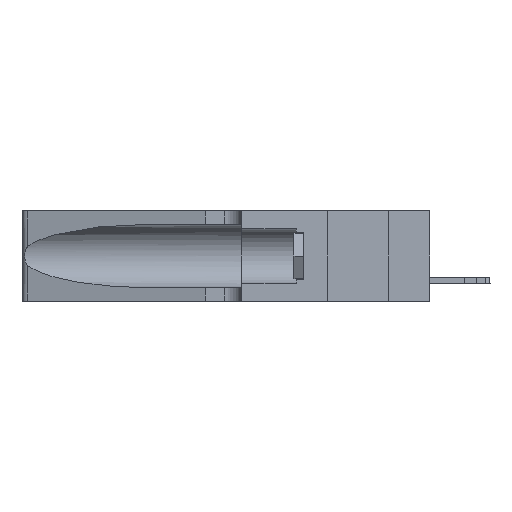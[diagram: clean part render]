
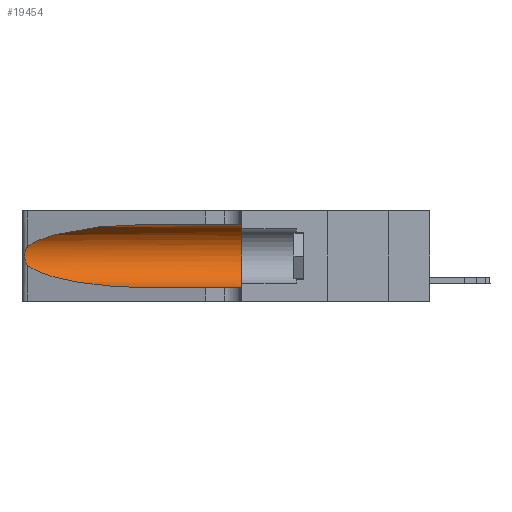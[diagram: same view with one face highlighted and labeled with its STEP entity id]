
A CAD part, left-side view. The second image highlights one B-rep face of the part: STEP entity #19454.
In plain terms, the highlighted cylindrical face has radius 3.308 mm (diameter 6.617 mm), a partial arc.
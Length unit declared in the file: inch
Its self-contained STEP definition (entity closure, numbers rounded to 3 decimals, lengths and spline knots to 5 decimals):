
#487 = ORIENTED_EDGE ( 'NONE', *, *, #19606, .T. ) ;
#594 = CARTESIAN_POINT ( 'NONE',  ( 0.1305, 0.72297, 0.05475 ) ) ;
#696 = CARTESIAN_POINT ( 'NONE',  ( 0.25854, 1.2359, 0.20912 ) ) ;
#829 = CARTESIAN_POINT ( 'NONE',  ( 0.25789, 1.23486, 0.15765 ) ) ;
#889 = CARTESIAN_POINT ( 'NONE',  ( 0.26075, 1.23896, 0.19203 ) ) ;
#1236 = DIRECTION ( 'NONE',  ( 0., -1., 0. ) ) ;
#1307 = DIRECTION ( 'NONE',  ( 0., 1., 0. ) ) ;
#1852 = EDGE_CURVE ( 'NONE', #2309, #6942, #5154, .T. ) ;
#2156 = EDGE_CURVE ( 'NONE', #19554, #5370, #11782, .T. ) ;
#2194 = CARTESIAN_POINT ( 'NONE',  ( 0.2373, 1.15595, 0.28018 ) ) ;
#2309 = VERTEX_POINT ( 'NONE', #5641 ) ;
#2811 = DIRECTION ( 'NONE',  ( 0., 0., -1. ) ) ;
#2937 = CARTESIAN_POINT ( 'NONE',  ( 0.25487, 1.22718, 0.14631 ) ) ;
#3590 = CARTESIAN_POINT ( 'NONE',  ( 0.25555, 1.22994, 0.2215 ) ) ;
#3851 = CARTESIAN_POINT ( 'NONE',  ( 0.26075, 1.23896, 0.178 ) ) ;
#3909 = VERTEX_POINT ( 'NONE', #14262 ) ;
#4840 = EDGE_LOOP ( 'NONE', ( #18273, #14750, #487, #16768, #6416, #5455 ) ) ;
#5136 = EDGE_CURVE ( 'NONE', #5370, #11224, #10935, .T. ) ;
#5154 = CIRCLE ( 'NONE', #13171, 0.13025 ) ;
#5287 = EDGE_CURVE ( 'NONE', #3909, #6942, #15941, .T. ) ;
#5370 = VERTEX_POINT ( 'NONE', #14126 ) ;
#5439 = CARTESIAN_POINT ( 'NONE',  ( 0.25787, 1.23484, 0.2124 ) ) ;
#5455 = ORIENTED_EDGE ( 'NONE', *, *, #14140, .F. ) ;
#5641 = CARTESIAN_POINT ( 'NONE',  ( 0.1305, 0.35, 0.31525 ) ) ;
#6026 = LINE ( 'NONE', #6101, #10466 ) ;
#6101 = CARTESIAN_POINT ( 'NONE',  ( 0.1305, 1.61858, 0.31525 ) ) ;
#6416 = ORIENTED_EDGE ( 'NONE', *, *, #1852, .F. ) ;
#6942 = VERTEX_POINT ( 'NONE', #18145 ) ;
#7665 = DIRECTION ( 'NONE',  ( 0., -1., 0. ) ) ;
#8390 = AXIS2_PLACEMENT_3D ( 'NONE', #10676, #1236, #2811 ) ;
#8391 = CARTESIAN_POINT ( 'NONE',  ( 0.18966, 0.96281, 0.31525 ) ) ;
#8731 = CARTESIAN_POINT ( 'NONE',  ( 0.1305, 0.72297, 0.31525 ) ) ;
#8964 = CARTESIAN_POINT ( 'NONE',  ( 0.1305, 0.35, 0.185 ) ) ;
#8981 = FACE_OUTER_BOUND ( 'NONE', #4840, .T. ) ;
#9329 = CARTESIAN_POINT ( 'NONE',  ( 0.1305, 1.61858, 0.05475 ) ) ;
#10265 = CARTESIAN_POINT ( 'NONE',  ( 0.25555, 1.22993, 0.14849 ) ) ;
#10466 = VECTOR ( 'NONE', #7665, 39.37008 ) ;
#10676 = CARTESIAN_POINT ( 'NONE',  ( 0.1305, 1.61858, 0.185 ) ) ;
#10935 = B_SPLINE_CURVE_WITH_KNOTS ( 'NONE', 3,
 ( #12938, #3590, #16096, #5439, #696, #14846, #889, #3851, #19593, #11866, #829, #16279, #10265, #16410 ),
 .UNSPECIFIED., .F., .F.,
 ( 4, 2, 2, 2, 2, 2, 4 ),
 ( 0., 0.00027, 0.00053, 0.00107, 0.0016, 0.00187, 0.00214 ),
 .UNSPECIFIED. ) ;
#11224 = VERTEX_POINT ( 'NONE', #2937 ) ;
#11733 = CARTESIAN_POINT ( 'NONE',  ( 0.1305, 0.72297, 0.31525 ) ) ;
#11782 =( BOUNDED_CURVE ( )  B_SPLINE_CURVE ( 3, ( #11733, #8391, #2194, #13279 ),
 .UNSPECIFIED., .F., .F. ) 
 B_SPLINE_CURVE_WITH_KNOTS ( ( 4, 4 ),
 ( 1.5708, 2.84003 ),
 .UNSPECIFIED. ) 
 CURVE ( )  GEOMETRIC_REPRESENTATION_ITEM ( )  RATIONAL_B_SPLINE_CURVE ( ( 1., 0.87, 0.87, 1. ) ) 
 REPRESENTATION_ITEM ( '' )  );
#11795 = VECTOR ( 'NONE', #18396, 39.37008 ) ;
#11866 = CARTESIAN_POINT ( 'NONE',  ( 0.25856, 1.23593, 0.16098 ) ) ;
#12134 =( BOUNDED_CURVE ( )  B_SPLINE_CURVE ( 3, ( #14489, #15865, #12661, #594 ),
 .UNSPECIFIED., .F., .F. ) 
 B_SPLINE_CURVE_WITH_KNOTS ( ( 4, 4 ),
 ( 3.44316, 4.71239 ),
 .UNSPECIFIED. ) 
 CURVE ( )  GEOMETRIC_REPRESENTATION_ITEM ( )  RATIONAL_B_SPLINE_CURVE ( ( 1., 0.87, 0.87, 1. ) ) 
 REPRESENTATION_ITEM ( '' )  );
#12274 = DIRECTION ( 'NONE',  ( 0., 0., 1. ) ) ;
#12661 = CARTESIAN_POINT ( 'NONE',  ( 0.18966, 0.96281, 0.05475 ) ) ;
#12938 = CARTESIAN_POINT ( 'NONE',  ( 0.25487, 1.22718, 0.22369 ) ) ;
#13097 = CYLINDRICAL_SURFACE ( 'NONE', #8390, 0.13025 ) ;
#13171 = AXIS2_PLACEMENT_3D ( 'NONE', #8964, #1307, #12274 ) ;
#13279 = CARTESIAN_POINT ( 'NONE',  ( 0.25487, 1.22718, 0.22369 ) ) ;
#14126 = CARTESIAN_POINT ( 'NONE',  ( 0.25487, 1.22718, 0.22369 ) ) ;
#14140 = EDGE_CURVE ( 'NONE', #19554, #2309, #6026, .T. ) ;
#14262 = CARTESIAN_POINT ( 'NONE',  ( 0.1305, 0.72297, 0.05475 ) ) ;
#14489 = CARTESIAN_POINT ( 'NONE',  ( 0.25487, 1.22718, 0.14631 ) ) ;
#14750 = ORIENTED_EDGE ( 'NONE', *, *, #5136, .T. ) ;
#14846 = CARTESIAN_POINT ( 'NONE',  ( 0.26018, 1.23835, 0.19895 ) ) ;
#15865 = CARTESIAN_POINT ( 'NONE',  ( 0.2373, 1.15595, 0.08982 ) ) ;
#15941 = LINE ( 'NONE', #9329, #11795 ) ;
#16096 = CARTESIAN_POINT ( 'NONE',  ( 0.25639, 1.23184, 0.21858 ) ) ;
#16279 = CARTESIAN_POINT ( 'NONE',  ( 0.25639, 1.23186, 0.15144 ) ) ;
#16410 = CARTESIAN_POINT ( 'NONE',  ( 0.25487, 1.22718, 0.14631 ) ) ;
#16768 = ORIENTED_EDGE ( 'NONE', *, *, #5287, .T. ) ;
#18145 = CARTESIAN_POINT ( 'NONE',  ( 0.1305, 0.35, 0.05475 ) ) ;
#18273 = ORIENTED_EDGE ( 'NONE', *, *, #2156, .T. ) ;
#18396 = DIRECTION ( 'NONE',  ( 0., -1., 0. ) ) ;
#19454 = ADVANCED_FACE ( 'NONE', ( #8981 ), #13097, .F. ) ;
#19554 = VERTEX_POINT ( 'NONE', #8731 ) ;
#19593 = CARTESIAN_POINT ( 'NONE',  ( 0.26017, 1.23833, 0.17102 ) ) ;
#19606 = EDGE_CURVE ( 'NONE', #11224, #3909, #12134, .T. ) ;
